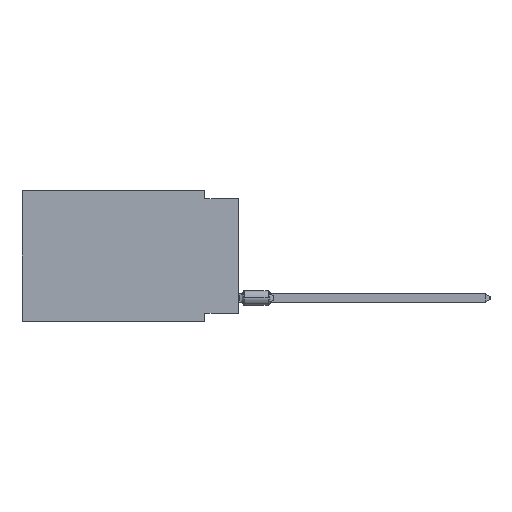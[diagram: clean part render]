
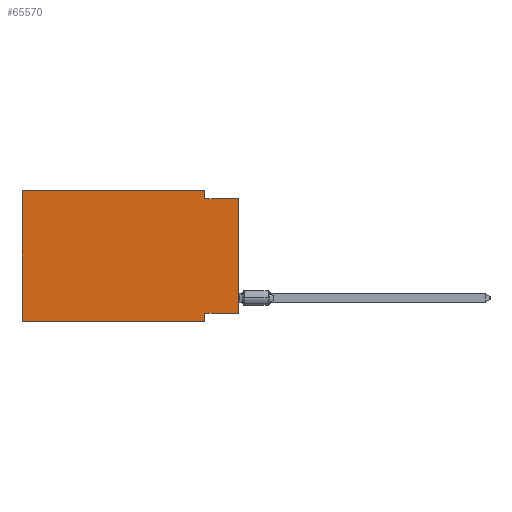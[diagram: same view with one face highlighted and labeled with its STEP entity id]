
A CAD part, left-side view. The second image highlights one B-rep face of the part: STEP entity #65570.
In plain terms, the highlighted planar face has unit normal (-1, 0, 0).
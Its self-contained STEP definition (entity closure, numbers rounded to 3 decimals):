
#1367 = VERTEX_POINT ( 'NONE', #9353 ) ;
#2582 = EDGE_CURVE ( 'NONE', #31955, #51829, #69636, .T. ) ;
#3594 = ORIENTED_EDGE ( 'NONE', *, *, #71963, .F. ) ;
#3883 = ORIENTED_EDGE ( 'NONE', *, *, #28051, .F. ) ;
#4949 = DIRECTION ( 'NONE',  ( 0., 0., -1. ) ) ;
#4969 = VECTOR ( 'NONE', #23675, 1000. ) ;
#5376 = CARTESIAN_POINT ( 'NONE',  ( 0., 16.383, 0. ) ) ;
#5438 = LINE ( 'NONE', #38047, #58239 ) ;
#7449 = CARTESIAN_POINT ( 'NONE',  ( 0., 16.383, 0. ) ) ;
#9353 = CARTESIAN_POINT ( 'NONE',  ( 0., 0., -9.271 ) ) ;
#9495 = CARTESIAN_POINT ( 'NONE',  ( 0., 2.54, -0.635 ) ) ;
#10014 = CARTESIAN_POINT ( 'NONE',  ( 0., 16.383, -9.906 ) ) ;
#10260 = VECTOR ( 'NONE', #37798, 1000. ) ;
#11976 = LINE ( 'NONE', #31191, #4969 ) ;
#12588 = VECTOR ( 'NONE', #23853, 1000. ) ;
#16996 = CARTESIAN_POINT ( 'NONE',  ( 0., 0., -0.635 ) ) ;
#17807 = EDGE_CURVE ( 'NONE', #1367, #61210, #54508, .T. ) ;
#18118 = DIRECTION ( 'NONE',  ( 0., 1., 0. ) ) ;
#19721 = VERTEX_POINT ( 'NONE', #10014 ) ;
#23675 = DIRECTION ( 'NONE',  ( 0., 0., -1. ) ) ;
#23679 = CARTESIAN_POINT ( 'NONE',  ( 0., 2.54, -9.906 ) ) ;
#23853 = DIRECTION ( 'NONE',  ( 0., 0., 1. ) ) ;
#24096 = CARTESIAN_POINT ( 'NONE',  ( 0., 16.383, 0. ) ) ;
#24151 = PLANE ( 'NONE',  #24618 ) ;
#24220 = VERTEX_POINT ( 'NONE', #9495 ) ;
#24328 = VERTEX_POINT ( 'NONE', #23679 ) ;
#24567 = CARTESIAN_POINT ( 'NONE',  ( 0., 16.383, 0. ) ) ;
#24618 = AXIS2_PLACEMENT_3D ( 'NONE', #24567, #63431, #4949 ) ;
#25231 = CARTESIAN_POINT ( 'NONE',  ( 0., 0., -0.635 ) ) ;
#27266 = VECTOR ( 'NONE', #68396, 1000. ) ;
#27506 = ORIENTED_EDGE ( 'NONE', *, *, #17807, .F. ) ;
#28051 = EDGE_CURVE ( 'NONE', #51829, #24220, #11976, .T. ) ;
#28392 = ORIENTED_EDGE ( 'NONE', *, *, #37807, .T. ) ;
#30847 = VECTOR ( 'NONE', #36545, 1000. ) ;
#31191 = CARTESIAN_POINT ( 'NONE',  ( 0., 2.54, 0. ) ) ;
#31955 = VERTEX_POINT ( 'NONE', #5376 ) ;
#33051 = CARTESIAN_POINT ( 'NONE',  ( 0., 2.54, 0. ) ) ;
#35193 = ORIENTED_EDGE ( 'NONE', *, *, #72691, .T. ) ;
#36230 = LINE ( 'NONE', #25231, #10260 ) ;
#36412 = LINE ( 'NONE', #76077, #12588 ) ;
#36545 = DIRECTION ( 'NONE',  ( 0., -1., 0. ) ) ;
#37798 = DIRECTION ( 'NONE',  ( 0., -1., 0. ) ) ;
#37807 = EDGE_CURVE ( 'NONE', #1367, #45768, #36412, .T. ) ;
#38047 = CARTESIAN_POINT ( 'NONE',  ( 0., 2.54, -9.906 ) ) ;
#41073 = EDGE_CURVE ( 'NONE', #61210, #24328, #5438, .T. ) ;
#42986 = FACE_OUTER_BOUND ( 'NONE', #48925, .T. ) ;
#45768 = VERTEX_POINT ( 'NONE', #16996 ) ;
#47670 = ORIENTED_EDGE ( 'NONE', *, *, #41073, .F. ) ;
#48087 = VECTOR ( 'NONE', #75680, 1000. ) ;
#48246 = CARTESIAN_POINT ( 'NONE',  ( 0., 0., -9.271 ) ) ;
#48251 = CARTESIAN_POINT ( 'NONE',  ( 0., 16.383, -9.906 ) ) ;
#48925 = EDGE_LOOP ( 'NONE', ( #28392, #73226, #3883, #68867, #3594, #35193, #47670, #27506 ) ) ;
#49793 = LINE ( 'NONE', #7449, #48087 ) ;
#51829 = VERTEX_POINT ( 'NONE', #33051 ) ;
#53991 = EDGE_CURVE ( 'NONE', #24220, #45768, #36230, .T. ) ;
#54508 = LINE ( 'NONE', #48246, #75422 ) ;
#56846 = DIRECTION ( 'NONE',  ( 0., 0., -1. ) ) ;
#58239 = VECTOR ( 'NONE', #56846, 1000. ) ;
#61210 = VERTEX_POINT ( 'NONE', #61775 ) ;
#61775 = CARTESIAN_POINT ( 'NONE',  ( 0., 2.54, -9.271 ) ) ;
#63431 = DIRECTION ( 'NONE',  ( 1., 0., 0. ) ) ;
#65570 = ADVANCED_FACE ( 'NONE', ( #42986 ), #24151, .F. ) ;
#68396 = DIRECTION ( 'NONE',  ( 0., -1., 0. ) ) ;
#68867 = ORIENTED_EDGE ( 'NONE', *, *, #2582, .F. ) ;
#69636 = LINE ( 'NONE', #24096, #27266 ) ;
#71963 = EDGE_CURVE ( 'NONE', #19721, #31955, #49793, .T. ) ;
#72691 = EDGE_CURVE ( 'NONE', #19721, #24328, #73305, .T. ) ;
#73226 = ORIENTED_EDGE ( 'NONE', *, *, #53991, .F. ) ;
#73305 = LINE ( 'NONE', #48251, #30847 ) ;
#75422 = VECTOR ( 'NONE', #18118, 1000. ) ;
#75680 = DIRECTION ( 'NONE',  ( 0., 0., 1. ) ) ;
#76077 = CARTESIAN_POINT ( 'NONE',  ( 0., 0., 0. ) ) ;
